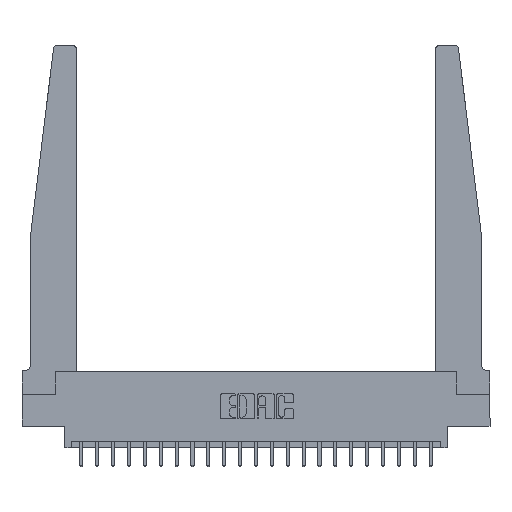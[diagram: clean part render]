
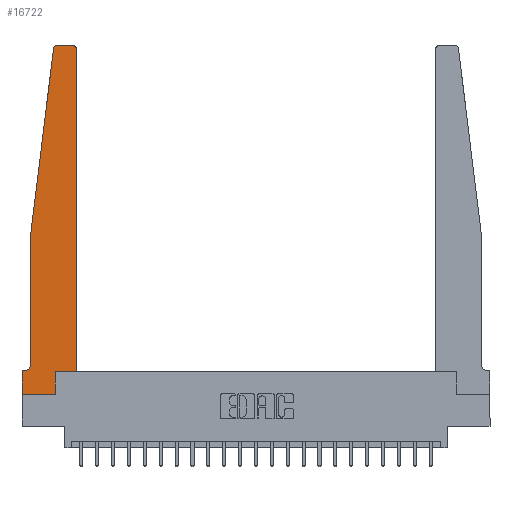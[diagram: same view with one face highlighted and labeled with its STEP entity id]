
A CAD part, top view. The second image highlights one B-rep face of the part: STEP entity #16722.
In plain terms, the highlighted planar face has unit normal (0, 0, 1).
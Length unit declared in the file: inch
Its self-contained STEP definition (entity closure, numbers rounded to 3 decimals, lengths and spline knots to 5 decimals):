
#410 = CARTESIAN_POINT ( 'NONE',  ( 0.2605, 0.18, 0.37 ) ) ;
#659 = AXIS2_PLACEMENT_3D ( 'NONE', #19820, #17764, #1856 ) ;
#770 = CARTESIAN_POINT ( 'NONE',  ( 0.425, 0.18, 0.37 ) ) ;
#1352 = EDGE_CURVE ( 'NONE', #1440, #21478, #11183, .T. ) ;
#1374 = ORIENTED_EDGE ( 'NONE', *, *, #15227, .T. ) ;
#1389 = LINE ( 'NONE', #15205, #6464 ) ;
#1440 = VERTEX_POINT ( 'NONE', #22079 ) ;
#1578 = EDGE_CURVE ( 'NONE', #17427, #17063, #22776, .T. ) ;
#1666 = VECTOR ( 'NONE', #19028, 39.37008 ) ;
#1800 = VECTOR ( 'NONE', #11873, 39.37008 ) ;
#1856 = DIRECTION ( 'NONE',  ( 1., 0., 0. ) ) ;
#2187 = CARTESIAN_POINT ( 'NONE',  ( 0.2605, 0., 0.37 ) ) ;
#2300 = FACE_OUTER_BOUND ( 'NONE', #2992, .T. ) ;
#2324 = EDGE_CURVE ( 'NONE', #17572, #15895, #21673, .T. ) ;
#2453 = AXIS2_PLACEMENT_3D ( 'NONE', #7651, #10917, #12664 ) ;
#2992 = EDGE_LOOP ( 'NONE', ( #4748, #5065, #20942, #18965, #1374, #11249, #5412, #18226, #12870, #7987, #21418, #16159 ) ) ;
#3098 = EDGE_CURVE ( 'NONE', #17063, #10633, #3523, .T. ) ;
#3285 = AXIS2_PLACEMENT_3D ( 'NONE', #7841, #15459, #14916 ) ;
#3523 = CIRCLE ( 'NONE', #17188, 0.03 ) ;
#3729 = VERTEX_POINT ( 'NONE', #2187 ) ;
#4041 = PLANE ( 'NONE',  #659 ) ;
#4463 = CARTESIAN_POINT ( 'NONE',  ( 0.065, 0.2375, 0.37 ) ) ;
#4541 = DIRECTION ( 'NONE',  ( 1., 0., 0. ) ) ;
#4696 = CARTESIAN_POINT ( 'NONE',  ( 0.395, 2.75, 0.37 ) ) ;
#4748 = ORIENTED_EDGE ( 'NONE', *, *, #18029, .T. ) ;
#4983 = DIRECTION ( 'NONE',  ( 0., -1., 0. ) ) ;
#4996 = CARTESIAN_POINT ( 'NONE',  ( 0.25, 2.75, 0.37 ) ) ;
#5065 = ORIENTED_EDGE ( 'NONE', *, *, #17432, .T. ) ;
#5145 = CARTESIAN_POINT ( 'NONE',  ( 0.015, 0.1875, 0.37 ) ) ;
#5412 = ORIENTED_EDGE ( 'NONE', *, *, #22346, .T. ) ;
#5918 = VERTEX_POINT ( 'NONE', #13381 ) ;
#6464 = VECTOR ( 'NONE', #4983, 39.37008 ) ;
#6844 = DIRECTION ( 'NONE',  ( 1., 0., 0. ) ) ;
#7085 = LINE ( 'NONE', #4996, #19588 ) ;
#7123 = CARTESIAN_POINT ( 'NONE',  ( 0.065, 1.25, 0.37 ) ) ;
#7468 = CARTESIAN_POINT ( 'NONE',  ( 0., 0.1875, 0.37 ) ) ;
#7651 = CARTESIAN_POINT ( 'NONE',  ( 0.015, 0.2375, 0.37 ) ) ;
#7841 = CARTESIAN_POINT ( 'NONE',  ( 0.27653, 2.72, 0.37 ) ) ;
#7957 = VERTEX_POINT ( 'NONE', #4463 ) ;
#7987 = ORIENTED_EDGE ( 'NONE', *, *, #18559, .T. ) ;
#8147 = VECTOR ( 'NONE', #4541, 39.37008 ) ;
#8586 = LINE ( 'NONE', #15663, #17899 ) ;
#8952 = CARTESIAN_POINT ( 'NONE',  ( 0.395, 2.72, 0.37 ) ) ;
#9885 = DIRECTION ( 'NONE',  ( -0.122, -0.992, 0. ) ) ;
#10349 = EDGE_CURVE ( 'NONE', #21478, #7957, #1389, .T. ) ;
#10356 = EDGE_CURVE ( 'NONE', #3729, #19837, #20534, .T. ) ;
#10633 = VERTEX_POINT ( 'NONE', #4696 ) ;
#10917 = DIRECTION ( 'NONE',  ( 0., 0., -1. ) ) ;
#11183 = LINE ( 'NONE', #18722, #19945 ) ;
#11249 = ORIENTED_EDGE ( 'NONE', *, *, #2324, .T. ) ;
#11605 = CARTESIAN_POINT ( 'NONE',  ( 0.2605, 0.18, 0.37 ) ) ;
#11683 = EDGE_CURVE ( 'NONE', #5918, #3729, #8586, .T. ) ;
#11873 = DIRECTION ( 'NONE',  ( 0., 1., 0. ) ) ;
#12086 = VERTEX_POINT ( 'NONE', #17149 ) ;
#12471 = CIRCLE ( 'NONE', #2453, 0.05 ) ;
#12664 = DIRECTION ( 'NONE',  ( -1., 0., 0. ) ) ;
#12870 = ORIENTED_EDGE ( 'NONE', *, *, #10356, .T. ) ;
#13381 = CARTESIAN_POINT ( 'NONE',  ( 0., 0., 0.37 ) ) ;
#14043 = DIRECTION ( 'NONE',  ( -1., 0., 0. ) ) ;
#14061 = DIRECTION ( 'NONE',  ( 0., 0., 1. ) ) ;
#14351 = VECTOR ( 'NONE', #15536, 39.37008 ) ;
#14435 = VECTOR ( 'NONE', #14701, 39.37008 ) ;
#14701 = DIRECTION ( 'NONE',  ( -1., 0., 0. ) ) ;
#14916 = DIRECTION ( 'NONE',  ( 1., 0., 0. ) ) ;
#15205 = CARTESIAN_POINT ( 'NONE',  ( 0.065, 1.25, 0.37 ) ) ;
#15227 = EDGE_CURVE ( 'NONE', #7957, #17572, #12471, .T. ) ;
#15459 = DIRECTION ( 'NONE',  ( 0., 0., 1. ) ) ;
#15536 = DIRECTION ( 'NONE',  ( 0., -1., 0. ) ) ;
#15663 = CARTESIAN_POINT ( 'NONE',  ( 0., 0., 0.37 ) ) ;
#15895 = VERTEX_POINT ( 'NONE', #7468 ) ;
#16159 = ORIENTED_EDGE ( 'NONE', *, *, #3098, .T. ) ;
#16722 = ADVANCED_FACE ( 'NONE', ( #2300 ), #4041, .T. ) ;
#17063 = VERTEX_POINT ( 'NONE', #19238 ) ;
#17149 = CARTESIAN_POINT ( 'NONE',  ( 0.27653, 2.75, 0.37 ) ) ;
#17164 = LINE ( 'NONE', #19020, #14351 ) ;
#17188 = AXIS2_PLACEMENT_3D ( 'NONE', #8952, #14061, #21141 ) ;
#17364 = CIRCLE ( 'NONE', #3285, 0.03 ) ;
#17427 = VERTEX_POINT ( 'NONE', #770 ) ;
#17432 = EDGE_CURVE ( 'NONE', #12086, #1440, #17364, .T. ) ;
#17572 = VERTEX_POINT ( 'NONE', #5145 ) ;
#17764 = DIRECTION ( 'NONE',  ( 0., 0., 1. ) ) ;
#17899 = VECTOR ( 'NONE', #6844, 39.37008 ) ;
#18029 = EDGE_CURVE ( 'NONE', #10633, #12086, #7085, .T. ) ;
#18226 = ORIENTED_EDGE ( 'NONE', *, *, #11683, .T. ) ;
#18299 = CARTESIAN_POINT ( 'NONE',  ( 0.065, 0.1875, 0.37 ) ) ;
#18559 = EDGE_CURVE ( 'NONE', #19837, #17427, #18698, .T. ) ;
#18698 = LINE ( 'NONE', #20890, #8147 ) ;
#18722 = CARTESIAN_POINT ( 'NONE',  ( 0.065, 1.25, 0.37 ) ) ;
#18965 = ORIENTED_EDGE ( 'NONE', *, *, #10349, .T. ) ;
#19020 = CARTESIAN_POINT ( 'NONE',  ( 0., 0., 0.37 ) ) ;
#19028 = DIRECTION ( 'NONE',  ( 0., 1., 0. ) ) ;
#19238 = CARTESIAN_POINT ( 'NONE',  ( 0.425, 2.72, 0.37 ) ) ;
#19588 = VECTOR ( 'NONE', #14043, 39.37008 ) ;
#19820 = CARTESIAN_POINT ( 'NONE',  ( 0., 0.1875, 0.37 ) ) ;
#19837 = VERTEX_POINT ( 'NONE', #410 ) ;
#19945 = VECTOR ( 'NONE', #9885, 39.37008 ) ;
#20534 = LINE ( 'NONE', #11605, #1666 ) ;
#20890 = CARTESIAN_POINT ( 'NONE',  ( 0.425, 0.18, 0.37 ) ) ;
#20942 = ORIENTED_EDGE ( 'NONE', *, *, #1352, .T. ) ;
#21141 = DIRECTION ( 'NONE',  ( 1., 0., 0. ) ) ;
#21418 = ORIENTED_EDGE ( 'NONE', *, *, #1578, .T. ) ;
#21478 = VERTEX_POINT ( 'NONE', #7123 ) ;
#21673 = LINE ( 'NONE', #18299, #14435 ) ;
#22079 = CARTESIAN_POINT ( 'NONE',  ( 0.24675, 2.72367, 0.37 ) ) ;
#22320 = CARTESIAN_POINT ( 'NONE',  ( 0.425, 0.18, 0.37 ) ) ;
#22346 = EDGE_CURVE ( 'NONE', #15895, #5918, #17164, .T. ) ;
#22776 = LINE ( 'NONE', #22320, #1800 ) ;
